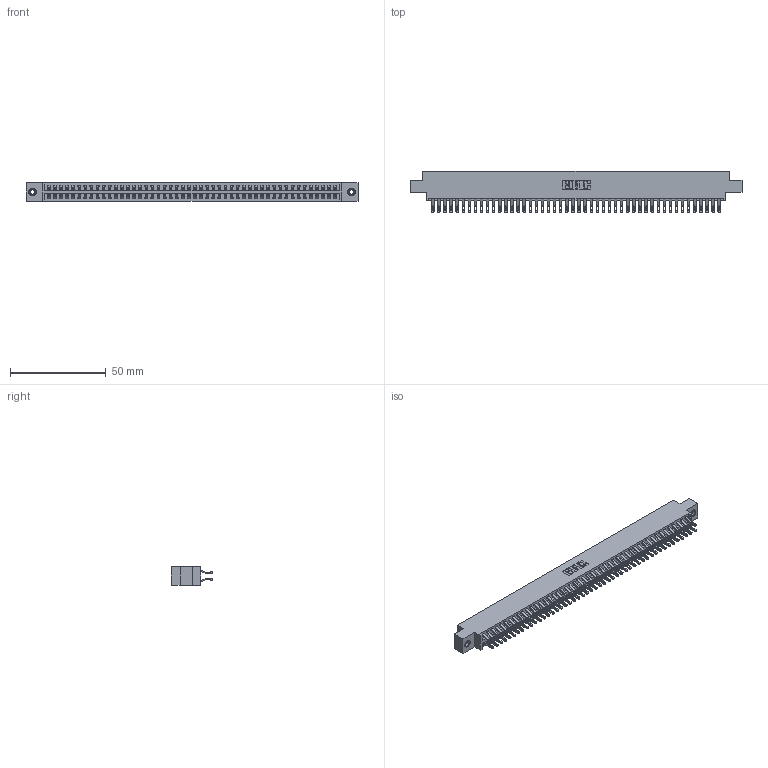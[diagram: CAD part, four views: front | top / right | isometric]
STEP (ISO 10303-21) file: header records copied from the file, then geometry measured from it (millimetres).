
FILE_DESCRIPTION (( 'STEP AP203' ), '1' );
FILE_NAME ('396-096-555-808.STEP', '2019-11-02T16:48:16', ( '' ), ( '' ), 'SwSTEP 2.0', 'SolidWorks 2016', '' );
FILE_SCHEMA (( 'CONFIG_CONTROL_DESIGN' ));
Length unit declared in the file: inch
Products named in the file (4): 345-292-001_555 Tail; 345-250-001_345-250-003-102; 396-096-555-808; 346 Part_0.170 Offset - 0.156 Dia-TI
Assembly tree (99 placements, depth 2):
  396-096-555-808
    346 Part_0.170 Offset - 0.156 Dia-TI
    345-292-001_555 Tail  x96
    345-250-001_345-250-003-102  x2
Bounding box: 172.97 x 21.46 x 9.4 mm (x, y, z)
Volume: 17031 mm3; surface area: 24696.8 mm2
Topology: 99 solids, 99 shells, 5754 faces, 18045 edges, 12022 vertices
Faces by surface type: plane 3280, cylinder 2458, cone 12, torus 4
Entity records: 32162 total; most frequent: CARTESIAN_POINT 5313, ORIENTED_EDGE 5210, DIRECTION 4727, EDGE_CURVE 2605, VECTOR 2241, LINE 2241, VERTEX_POINT 1732, AXIS2_PLACEMENT_3D 1243
